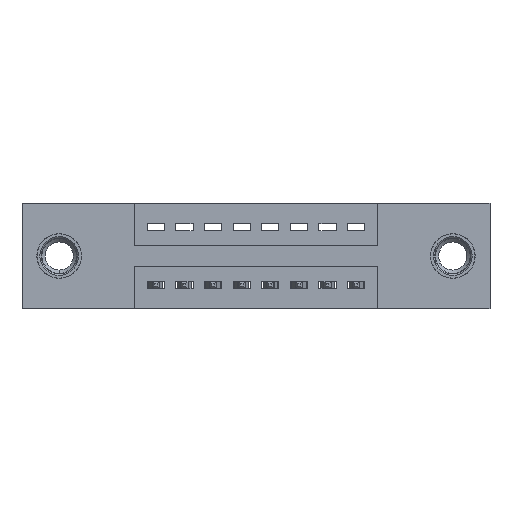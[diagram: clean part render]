
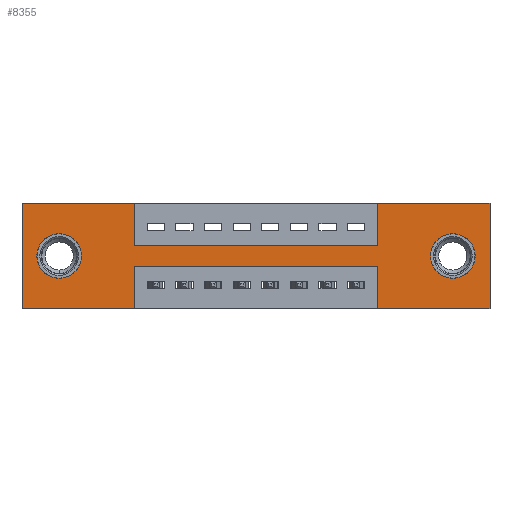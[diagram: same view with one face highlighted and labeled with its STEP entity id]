
A CAD part, front view. The second image highlights one B-rep face of the part: STEP entity #8355.
In plain terms, the highlighted planar face has unit normal (0, -1, 0).
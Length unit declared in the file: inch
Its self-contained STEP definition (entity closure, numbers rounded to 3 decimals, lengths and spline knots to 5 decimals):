
#17 = DIRECTION ( 'NONE',  ( 0., 0., -1. ) ) ;
#121 = EDGE_CURVE ( 'NONE', #8469, #9040, #149, .T. ) ;
#149 = LINE ( 'NONE', #6508, #11562 ) ;
#317 = EDGE_CURVE ( 'NONE', #1537, #7055, #8865, .T. ) ;
#340 = CARTESIAN_POINT ( 'NONE',  ( 0.13, 0., -0.185 ) ) ;
#353 = VERTEX_POINT ( 'NONE', #5007 ) ;
#497 = EDGE_CURVE ( 'NONE', #7380, #4653, #6729, .T. ) ;
#554 = CIRCLE ( 'NONE', #1608, 0.078 ) ;
#670 = EDGE_CURVE ( 'NONE', #4921, #7380, #1989, .T. ) ;
#738 = VERTEX_POINT ( 'NONE', #4534 ) ;
#885 = LINE ( 'NONE', #3696, #1893 ) ;
#896 = CARTESIAN_POINT ( 'NONE',  ( 1.505, 0., -0.185 ) ) ;
#928 = DIRECTION ( 'NONE',  ( 1., 0., 0. ) ) ;
#979 = CARTESIAN_POINT ( 'NONE',  ( 0.3925, 0., -0.15 ) ) ;
#1018 = CARTESIAN_POINT ( 'NONE',  ( 0.3925, 0., 0. ) ) ;
#1022 = ORIENTED_EDGE ( 'NONE', *, *, #9159, .F. ) ;
#1107 = CARTESIAN_POINT ( 'NONE',  ( 1.2425, 0., -0.37 ) ) ;
#1307 = CIRCLE ( 'NONE', #7649, 0.078 ) ;
#1333 = CARTESIAN_POINT ( 'NONE',  ( 1.2425, 0., -0.37 ) ) ;
#1334 = LINE ( 'NONE', #5618, #1609 ) ;
#1361 = CARTESIAN_POINT ( 'NONE',  ( 0.13, 0., -0.107 ) ) ;
#1537 = VERTEX_POINT ( 'NONE', #1333 ) ;
#1608 = AXIS2_PLACEMENT_3D ( 'NONE', #8224, #3754, #1740 ) ;
#1609 = VECTOR ( 'NONE', #3727, 39.37008 ) ;
#1740 = DIRECTION ( 'NONE',  ( 0., 0., -1. ) ) ;
#1816 = ORIENTED_EDGE ( 'NONE', *, *, #670, .F. ) ;
#1856 = FACE_BOUND ( 'NONE', #10708, .T. ) ;
#1893 = VECTOR ( 'NONE', #11759, 39.37008 ) ;
#1900 = VERTEX_POINT ( 'NONE', #3670 ) ;
#1989 = LINE ( 'NONE', #7942, #6856 ) ;
#2019 = DIRECTION ( 'NONE',  ( 0., 0., -1. ) ) ;
#2410 = ORIENTED_EDGE ( 'NONE', *, *, #7860, .T. ) ;
#2455 = DIRECTION ( 'NONE',  ( -1., 0., 0. ) ) ;
#2545 = LINE ( 'NONE', #2841, #9955 ) ;
#2629 = CARTESIAN_POINT ( 'NONE',  ( 1.505, 0., -0.263 ) ) ;
#2841 = CARTESIAN_POINT ( 'NONE',  ( 0.3925, 0., -0.22 ) ) ;
#2945 = CARTESIAN_POINT ( 'NONE',  ( 0., 0., -0.37 ) ) ;
#2972 = VERTEX_POINT ( 'NONE', #1361 ) ;
#3001 = CARTESIAN_POINT ( 'NONE',  ( 0.3925, 0., -0.37 ) ) ;
#3005 = ORIENTED_EDGE ( 'NONE', *, *, #7267, .T. ) ;
#3043 = VERTEX_POINT ( 'NONE', #4225 ) ;
#3045 = AXIS2_PLACEMENT_3D ( 'NONE', #896, #5407, #4448 ) ;
#3078 = ORIENTED_EDGE ( 'NONE', *, *, #4880, .F. ) ;
#3083 = VECTOR ( 'NONE', #5458, 39.37008 ) ;
#3199 = CARTESIAN_POINT ( 'NONE',  ( 0.3925, 0., -0.37 ) ) ;
#3282 = EDGE_CURVE ( 'NONE', #4653, #738, #6360, .T. ) ;
#3638 = CARTESIAN_POINT ( 'NONE',  ( 0.13, 0., -0.263 ) ) ;
#3670 = CARTESIAN_POINT ( 'NONE',  ( 0., 0., -0.37 ) ) ;
#3672 = AXIS2_PLACEMENT_3D ( 'NONE', #2945, #6613, #2019 ) ;
#3676 = EDGE_CURVE ( 'NONE', #1900, #3043, #6930, .T. ) ;
#3696 = CARTESIAN_POINT ( 'NONE',  ( 0., 0., 0. ) ) ;
#3727 = DIRECTION ( 'NONE',  ( -1., 0., 0. ) ) ;
#3754 = DIRECTION ( 'NONE',  ( 0., 1., 0. ) ) ;
#3792 = ORIENTED_EDGE ( 'NONE', *, *, #3676, .F. ) ;
#3911 = PLANE ( 'NONE',  #3672 ) ;
#4129 = LINE ( 'NONE', #4249, #4574 ) ;
#4225 = CARTESIAN_POINT ( 'NONE',  ( 0., 0., 0. ) ) ;
#4249 = CARTESIAN_POINT ( 'NONE',  ( 0., 0., -0.37 ) ) ;
#4448 = DIRECTION ( 'NONE',  ( 0., 0., -1. ) ) ;
#4534 = CARTESIAN_POINT ( 'NONE',  ( 1.2425, 0., 0. ) ) ;
#4574 = VECTOR ( 'NONE', #2455, 39.37008 ) ;
#4653 = VERTEX_POINT ( 'NONE', #6274 ) ;
#4749 = DIRECTION ( 'NONE',  ( 0., 0., -1. ) ) ;
#4838 = DIRECTION ( 'NONE',  ( -1., 0., 0. ) ) ;
#4852 = ORIENTED_EDGE ( 'NONE', *, *, #121, .F. ) ;
#4880 = EDGE_CURVE ( 'NONE', #3043, #4921, #885, .T. ) ;
#4921 = VERTEX_POINT ( 'NONE', #1018 ) ;
#4983 = DIRECTION ( 'NONE',  ( 0., 0., 1. ) ) ;
#4994 = VECTOR ( 'NONE', #5399, 39.37008 ) ;
#5007 = CARTESIAN_POINT ( 'NONE',  ( 0.3925, 0., -0.22 ) ) ;
#5111 = VECTOR ( 'NONE', #4983, 39.37008 ) ;
#5187 = ORIENTED_EDGE ( 'NONE', *, *, #11437, .T. ) ;
#5268 = CARTESIAN_POINT ( 'NONE',  ( 0.3925, 0., -0.15 ) ) ;
#5399 = DIRECTION ( 'NONE',  ( 1., 0., 0. ) ) ;
#5407 = DIRECTION ( 'NONE',  ( 0., 1., 0. ) ) ;
#5458 = DIRECTION ( 'NONE',  ( 0., 0., 1. ) ) ;
#5584 = LINE ( 'NONE', #3001, #5719 ) ;
#5618 = CARTESIAN_POINT ( 'NONE',  ( 0., 0., -0.37 ) ) ;
#5719 = VECTOR ( 'NONE', #17, 39.37008 ) ;
#6014 = DIRECTION ( 'NONE',  ( 0., 0., 1. ) ) ;
#6274 = CARTESIAN_POINT ( 'NONE',  ( 1.2425, 0., -0.15 ) ) ;
#6358 = ORIENTED_EDGE ( 'NONE', *, *, #317, .F. ) ;
#6360 = LINE ( 'NONE', #10001, #3083 ) ;
#6475 = EDGE_CURVE ( 'NONE', #7912, #1900, #1334, .T. ) ;
#6508 = CARTESIAN_POINT ( 'NONE',  ( 1.635, 0., 0. ) ) ;
#6584 = DIRECTION ( 'NONE',  ( 0., 1., 0. ) ) ;
#6613 = DIRECTION ( 'NONE',  ( 0., -1., 0. ) ) ;
#6652 = ORIENTED_EDGE ( 'NONE', *, *, #3282, .F. ) ;
#6729 = LINE ( 'NONE', #979, #10682 ) ;
#6856 = VECTOR ( 'NONE', #9740, 39.37008 ) ;
#6930 = LINE ( 'NONE', #10459, #5111 ) ;
#6988 = EDGE_CURVE ( 'NONE', #7555, #7600, #11723, .T. ) ;
#7036 = AXIS2_PLACEMENT_3D ( 'NONE', #11316, #7782, #6014 ) ;
#7055 = VERTEX_POINT ( 'NONE', #7231 ) ;
#7231 = CARTESIAN_POINT ( 'NONE',  ( 1.2425, 0., -0.22 ) ) ;
#7267 = EDGE_CURVE ( 'NONE', #2972, #7572, #10007, .T. ) ;
#7380 = VERTEX_POINT ( 'NONE', #5268 ) ;
#7555 = VERTEX_POINT ( 'NONE', #10747 ) ;
#7572 = VERTEX_POINT ( 'NONE', #3638 ) ;
#7600 = VERTEX_POINT ( 'NONE', #2629 ) ;
#7649 = AXIS2_PLACEMENT_3D ( 'NONE', #340, #6584, #9419 ) ;
#7782 = DIRECTION ( 'NONE',  ( 0., 1., 0. ) ) ;
#7860 = EDGE_CURVE ( 'NONE', #7572, #2972, #1307, .T. ) ;
#7912 = VERTEX_POINT ( 'NONE', #3199 ) ;
#7942 = CARTESIAN_POINT ( 'NONE',  ( 0.3925, 0., 0. ) ) ;
#8207 = CARTESIAN_POINT ( 'NONE',  ( 1.635, 0., -0.37 ) ) ;
#8224 = CARTESIAN_POINT ( 'NONE',  ( 1.505, 0., -0.185 ) ) ;
#8355 = ADVANCED_FACE ( 'NONE', ( #11253, #1856, #10983 ), #3911, .T. ) ;
#8372 = EDGE_LOOP ( 'NONE', ( #8628, #5187 ) ) ;
#8452 = ORIENTED_EDGE ( 'NONE', *, *, #11796, .F. ) ;
#8469 = VERTEX_POINT ( 'NONE', #9474 ) ;
#8628 = ORIENTED_EDGE ( 'NONE', *, *, #6988, .T. ) ;
#8689 = ORIENTED_EDGE ( 'NONE', *, *, #6475, .F. ) ;
#8865 = LINE ( 'NONE', #1107, #10416 ) ;
#9040 = VERTEX_POINT ( 'NONE', #8207 ) ;
#9159 = EDGE_CURVE ( 'NONE', #7055, #353, #2545, .T. ) ;
#9419 = DIRECTION ( 'NONE',  ( 0., 0., 1. ) ) ;
#9474 = CARTESIAN_POINT ( 'NONE',  ( 1.635, 0., 0. ) ) ;
#9740 = DIRECTION ( 'NONE',  ( 0., 0., -1. ) ) ;
#9794 = ORIENTED_EDGE ( 'NONE', *, *, #10075, .F. ) ;
#9955 = VECTOR ( 'NONE', #4838, 39.37008 ) ;
#10001 = CARTESIAN_POINT ( 'NONE',  ( 1.2425, 0., 0. ) ) ;
#10007 = CIRCLE ( 'NONE', #7036, 0.078 ) ;
#10075 = EDGE_CURVE ( 'NONE', #9040, #1537, #4129, .T. ) ;
#10223 = EDGE_CURVE ( 'NONE', #738, #8469, #11634, .T. ) ;
#10416 = VECTOR ( 'NONE', #10995, 39.37008 ) ;
#10420 = EDGE_LOOP ( 'NONE', ( #8452, #1022, #6358, #9794, #4852, #11560, #6652, #11118, #1816, #3078, #3792, #8689 ) ) ;
#10459 = CARTESIAN_POINT ( 'NONE',  ( 0., 0., 0. ) ) ;
#10682 = VECTOR ( 'NONE', #928, 39.37008 ) ;
#10708 = EDGE_LOOP ( 'NONE', ( #3005, #2410 ) ) ;
#10747 = CARTESIAN_POINT ( 'NONE',  ( 1.505, 0., -0.107 ) ) ;
#10804 = CARTESIAN_POINT ( 'NONE',  ( 0., 0., 0. ) ) ;
#10983 = FACE_OUTER_BOUND ( 'NONE', #10420, .T. ) ;
#10995 = DIRECTION ( 'NONE',  ( 0., 0., 1. ) ) ;
#11118 = ORIENTED_EDGE ( 'NONE', *, *, #497, .F. ) ;
#11253 = FACE_BOUND ( 'NONE', #8372, .T. ) ;
#11316 = CARTESIAN_POINT ( 'NONE',  ( 0.13, 0., -0.185 ) ) ;
#11437 = EDGE_CURVE ( 'NONE', #7600, #7555, #554, .T. ) ;
#11560 = ORIENTED_EDGE ( 'NONE', *, *, #10223, .F. ) ;
#11562 = VECTOR ( 'NONE', #4749, 39.37008 ) ;
#11634 = LINE ( 'NONE', #10804, #4994 ) ;
#11723 = CIRCLE ( 'NONE', #3045, 0.078 ) ;
#11759 = DIRECTION ( 'NONE',  ( 1., 0., 0. ) ) ;
#11796 = EDGE_CURVE ( 'NONE', #353, #7912, #5584, .T. ) ;
